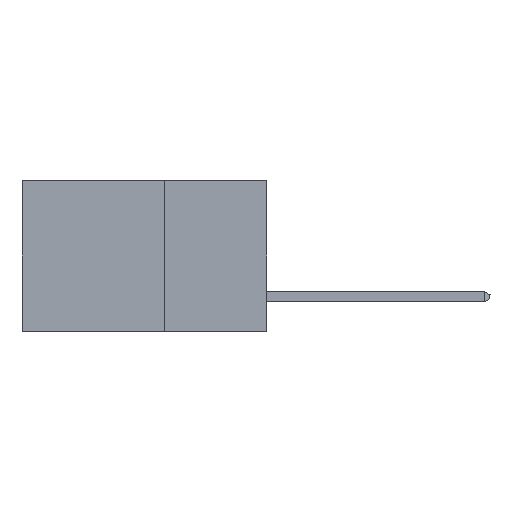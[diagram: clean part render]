
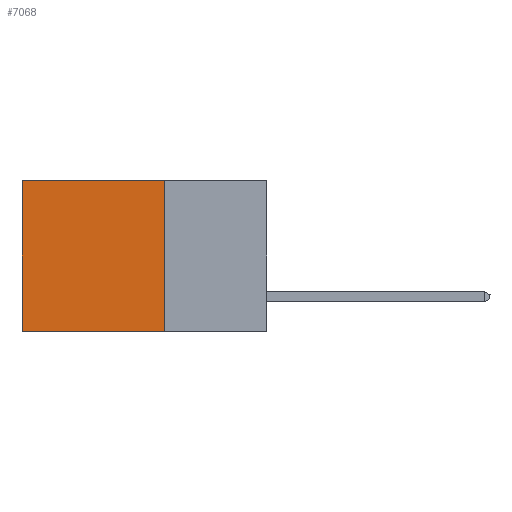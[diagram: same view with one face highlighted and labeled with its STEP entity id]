
A CAD part, left-side view. The second image highlights one B-rep face of the part: STEP entity #7068.
In plain terms, the highlighted planar face has unit normal (-1, 0, 0).
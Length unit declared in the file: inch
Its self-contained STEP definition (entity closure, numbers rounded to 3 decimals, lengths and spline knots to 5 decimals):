
#403 = CARTESIAN_POINT ( 'NONE',  ( 0.2875, 0.25, 0. ) ) ;
#1235 = DIRECTION ( 'NONE',  ( 0., 0., -1. ) ) ;
#1394 = EDGE_CURVE ( 'NONE', #7329, #30077, #28166, .T. ) ;
#2392 = DIRECTION ( 'NONE',  ( 0., 1., 0. ) ) ;
#3884 = DIRECTION ( 'NONE',  ( 0., 1., 0. ) ) ;
#4260 = EDGE_CURVE ( 'NONE', #7957, #25024, #37297, .T. ) ;
#7021 = EDGE_CURVE ( 'NONE', #30077, #25024, #35507, .T. ) ;
#7068 = ADVANCED_FACE ( 'NONE', ( #38557 ), #23878, .F. ) ;
#7329 = VERTEX_POINT ( 'NONE', #21170 ) ;
#7651 = AXIS2_PLACEMENT_3D ( 'NONE', #35310, #24271, #1235 ) ;
#7957 = VERTEX_POINT ( 'NONE', #24922 ) ;
#9518 = CARTESIAN_POINT ( 'NONE',  ( 0.2875, 0.6, 0. ) ) ;
#13145 = VECTOR ( 'NONE', #25124, 39.37008 ) ;
#13790 = ORIENTED_EDGE ( 'NONE', *, *, #15815, .T. ) ;
#14547 = CARTESIAN_POINT ( 'NONE',  ( 0.2875, 0.6, -0.37 ) ) ;
#15815 = EDGE_CURVE ( 'NONE', #7329, #7957, #22727, .T. ) ;
#16038 = VECTOR ( 'NONE', #2392, 39.37008 ) ;
#17041 = CARTESIAN_POINT ( 'NONE',  ( 0.2875, 0.25, -0.37 ) ) ;
#17215 = ORIENTED_EDGE ( 'NONE', *, *, #7021, .F. ) ;
#17840 = VECTOR ( 'NONE', #33850, 39.37008 ) ;
#21170 = CARTESIAN_POINT ( 'NONE',  ( 0.2875, 0.25, 0. ) ) ;
#21619 = EDGE_LOOP ( 'NONE', ( #28165, #17215, #25009, #13790 ) ) ;
#22727 = LINE ( 'NONE', #25959, #37869 ) ;
#23878 = PLANE ( 'NONE',  #7651 ) ;
#24271 = DIRECTION ( 'NONE',  ( 1., 0., 0. ) ) ;
#24922 = CARTESIAN_POINT ( 'NONE',  ( 0.2875, 0.6, 0. ) ) ;
#25009 = ORIENTED_EDGE ( 'NONE', *, *, #1394, .F. ) ;
#25024 = VERTEX_POINT ( 'NONE', #14547 ) ;
#25124 = DIRECTION ( 'NONE',  ( 0., 0., -1. ) ) ;
#25959 = CARTESIAN_POINT ( 'NONE',  ( 0.2875, 0.25, 0. ) ) ;
#26371 = CARTESIAN_POINT ( 'NONE',  ( 0.2875, 0.25, -0.37 ) ) ;
#28165 = ORIENTED_EDGE ( 'NONE', *, *, #4260, .T. ) ;
#28166 = LINE ( 'NONE', #403, #13145 ) ;
#30077 = VERTEX_POINT ( 'NONE', #17041 ) ;
#33850 = DIRECTION ( 'NONE',  ( 0., 0., -1. ) ) ;
#35310 = CARTESIAN_POINT ( 'NONE',  ( 0.2875, 0.25, 0. ) ) ;
#35507 = LINE ( 'NONE', #26371, #16038 ) ;
#37297 = LINE ( 'NONE', #9518, #17840 ) ;
#37869 = VECTOR ( 'NONE', #3884, 39.37008 ) ;
#38557 = FACE_OUTER_BOUND ( 'NONE', #21619, .T. ) ;
